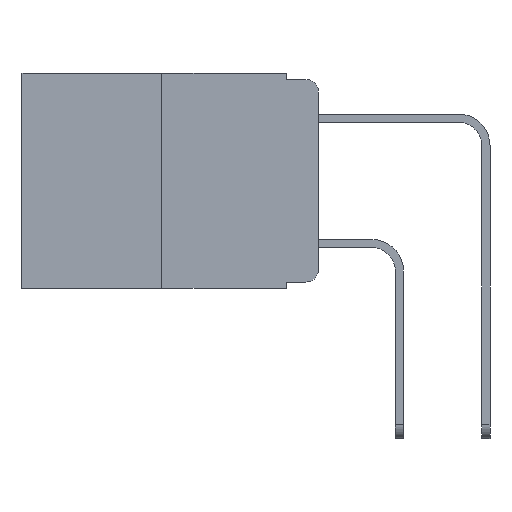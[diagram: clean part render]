
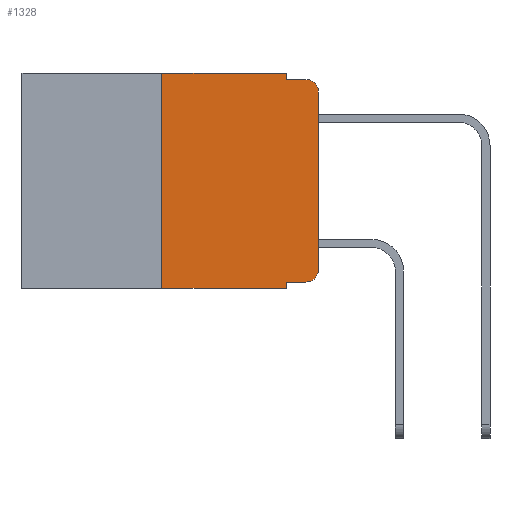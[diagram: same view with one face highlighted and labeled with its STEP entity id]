
A CAD part, left-side view. The second image highlights one B-rep face of the part: STEP entity #1328.
In plain terms, the highlighted planar face has unit normal (-1, 0, 0).
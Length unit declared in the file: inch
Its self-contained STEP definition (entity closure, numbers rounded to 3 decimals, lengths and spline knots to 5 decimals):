
#520 = ORIENTED_EDGE ( 'NONE', *, *, #11788, .F. ) ;
#544 = EDGE_CURVE ( 'NONE', #9214, #13852, #2338, .T. ) ;
#670 = VECTOR ( 'NONE', #9507, 39.37008 ) ;
#694 = VERTEX_POINT ( 'NONE', #13750 ) ;
#1055 = CARTESIAN_POINT ( 'NONE',  ( 0., 0.02, -0.01 ) ) ;
#1138 = DIRECTION ( 'NONE',  ( 1., 0., 0. ) ) ;
#1328 = ADVANCED_FACE ( 'NONE', ( #7653 ), #14650, .F. ) ;
#1337 = CARTESIAN_POINT ( 'NONE',  ( 0., 0.25, 0. ) ) ;
#1573 = DIRECTION ( 'NONE',  ( 0., 0., -1. ) ) ;
#1786 = CARTESIAN_POINT ( 'NONE',  ( 0., 0.051, 0. ) ) ;
#1998 = DIRECTION ( 'NONE',  ( 0., -1., 0. ) ) ;
#2338 = LINE ( 'NONE', #10830, #11243 ) ;
#2357 = DIRECTION ( 'NONE',  ( -1., 0., 0. ) ) ;
#3356 = VERTEX_POINT ( 'NONE', #3663 ) ;
#3663 = CARTESIAN_POINT ( 'NONE',  ( 0., 0.25, -0.343 ) ) ;
#3842 = VERTEX_POINT ( 'NONE', #1055 ) ;
#4135 = AXIS2_PLACEMENT_3D ( 'NONE', #9360, #2357, #10469 ) ;
#4154 = DIRECTION ( 'NONE',  ( 0., 0., -1. ) ) ;
#4188 = CIRCLE ( 'NONE', #4135, 0.02 ) ;
#4632 = VERTEX_POINT ( 'NONE', #11123 ) ;
#4668 = CIRCLE ( 'NONE', #6891, 0.02 ) ;
#4898 = CARTESIAN_POINT ( 'NONE',  ( 0., 0.051, -0.333 ) ) ;
#5058 = ORIENTED_EDGE ( 'NONE', *, *, #8766, .T. ) ;
#5104 = DIRECTION ( 'NONE',  ( 0., 0., -1. ) ) ;
#5173 = LINE ( 'NONE', #4898, #8303 ) ;
#5230 = CARTESIAN_POINT ( 'NONE',  ( 0., 0.051, -0.343 ) ) ;
#5750 = ORIENTED_EDGE ( 'NONE', *, *, #12557, .F. ) ;
#5844 = EDGE_CURVE ( 'NONE', #3356, #9050, #7983, .T. ) ;
#5989 = ORIENTED_EDGE ( 'NONE', *, *, #9495, .T. ) ;
#6007 = VECTOR ( 'NONE', #10457, 39.37008 ) ;
#6272 = CARTESIAN_POINT ( 'NONE',  ( 0., 0.051, 0. ) ) ;
#6308 = EDGE_LOOP ( 'NONE', ( #14989, #14837, #12925, #5750, #7150, #520, #11314, #9699, #5989, #5058 ) ) ;
#6375 = LINE ( 'NONE', #12728, #6007 ) ;
#6590 = CARTESIAN_POINT ( 'NONE',  ( 0., 0.02, -0.03 ) ) ;
#6629 = CARTESIAN_POINT ( 'NONE',  ( 0., 0.02, -0.333 ) ) ;
#6692 = CARTESIAN_POINT ( 'NONE',  ( 0., 0.051, -0.01 ) ) ;
#6784 = CARTESIAN_POINT ( 'NONE',  ( 0., 0., -0.313 ) ) ;
#6891 = AXIS2_PLACEMENT_3D ( 'NONE', #6590, #14556, #7760 ) ;
#7150 = ORIENTED_EDGE ( 'NONE', *, *, #12187, .F. ) ;
#7210 = CARTESIAN_POINT ( 'NONE',  ( 0., 0.051, -0.333 ) ) ;
#7417 = CARTESIAN_POINT ( 'NONE',  ( 0., 0.473, -0.343 ) ) ;
#7653 = FACE_OUTER_BOUND ( 'NONE', #6308, .T. ) ;
#7668 = VECTOR ( 'NONE', #1573, 39.37008 ) ;
#7760 = DIRECTION ( 'NONE',  ( 0., 0., -1. ) ) ;
#7983 = LINE ( 'NONE', #7417, #13660 ) ;
#8303 = VECTOR ( 'NONE', #8454, 39.37008 ) ;
#8454 = DIRECTION ( 'NONE',  ( 0., -1., 0. ) ) ;
#8766 = EDGE_CURVE ( 'NONE', #10829, #9214, #4188, .T. ) ;
#9050 = VERTEX_POINT ( 'NONE', #5230 ) ;
#9214 = VERTEX_POINT ( 'NONE', #6784 ) ;
#9360 = CARTESIAN_POINT ( 'NONE',  ( 0., 0.02, -0.313 ) ) ;
#9495 = EDGE_CURVE ( 'NONE', #11796, #10829, #5173, .T. ) ;
#9507 = DIRECTION ( 'NONE',  ( 0., 0., 1. ) ) ;
#9530 = VECTOR ( 'NONE', #4154, 39.37008 ) ;
#9699 = ORIENTED_EDGE ( 'NONE', *, *, #10253, .F. ) ;
#9987 = VECTOR ( 'NONE', #1998, 39.37008 ) ;
#9999 = LINE ( 'NONE', #1337, #670 ) ;
#10253 = EDGE_CURVE ( 'NONE', #11796, #9050, #12912, .T. ) ;
#10457 = DIRECTION ( 'NONE',  ( 0., -1., 0. ) ) ;
#10469 = DIRECTION ( 'NONE',  ( 0., 0., -1. ) ) ;
#10667 = LINE ( 'NONE', #6272, #7668 ) ;
#10680 = LINE ( 'NONE', #13576, #9987 ) ;
#10829 = VERTEX_POINT ( 'NONE', #6629 ) ;
#10830 = CARTESIAN_POINT ( 'NONE',  ( 0., 0., 0. ) ) ;
#11123 = CARTESIAN_POINT ( 'NONE',  ( 0., 0.25, 0. ) ) ;
#11243 = VECTOR ( 'NONE', #11751, 39.37008 ) ;
#11314 = ORIENTED_EDGE ( 'NONE', *, *, #5844, .T. ) ;
#11592 = CARTESIAN_POINT ( 'NONE',  ( 0., 0.473, 0. ) ) ;
#11751 = DIRECTION ( 'NONE',  ( 0., 0., 1. ) ) ;
#11788 = EDGE_CURVE ( 'NONE', #3356, #4632, #9999, .T. ) ;
#11796 = VERTEX_POINT ( 'NONE', #7210 ) ;
#12167 = VERTEX_POINT ( 'NONE', #6692 ) ;
#12187 = EDGE_CURVE ( 'NONE', #4632, #694, #10680, .T. ) ;
#12557 = EDGE_CURVE ( 'NONE', #694, #12167, #10667, .T. ) ;
#12728 = CARTESIAN_POINT ( 'NONE',  ( 0., 0.051, -0.01 ) ) ;
#12912 = LINE ( 'NONE', #1786, #9530 ) ;
#12925 = ORIENTED_EDGE ( 'NONE', *, *, #13305, .F. ) ;
#13109 = AXIS2_PLACEMENT_3D ( 'NONE', #11592, #1138, #5104 ) ;
#13305 = EDGE_CURVE ( 'NONE', #12167, #3842, #6375, .T. ) ;
#13576 = CARTESIAN_POINT ( 'NONE',  ( 0., 0.473, 0. ) ) ;
#13660 = VECTOR ( 'NONE', #14223, 39.37008 ) ;
#13750 = CARTESIAN_POINT ( 'NONE',  ( 0., 0.051, 0. ) ) ;
#13852 = VERTEX_POINT ( 'NONE', #14862 ) ;
#14223 = DIRECTION ( 'NONE',  ( 0., -1., 0. ) ) ;
#14556 = DIRECTION ( 'NONE',  ( -1., 0., 0. ) ) ;
#14650 = PLANE ( 'NONE',  #13109 ) ;
#14800 = EDGE_CURVE ( 'NONE', #13852, #3842, #4668, .T. ) ;
#14837 = ORIENTED_EDGE ( 'NONE', *, *, #14800, .T. ) ;
#14862 = CARTESIAN_POINT ( 'NONE',  ( 0., 0., -0.03 ) ) ;
#14989 = ORIENTED_EDGE ( 'NONE', *, *, #544, .T. ) ;
